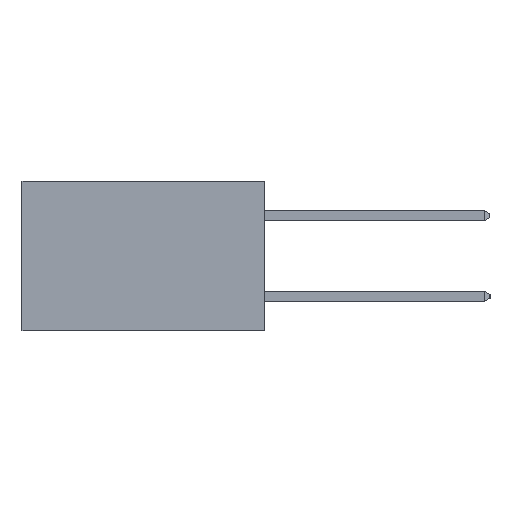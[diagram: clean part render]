
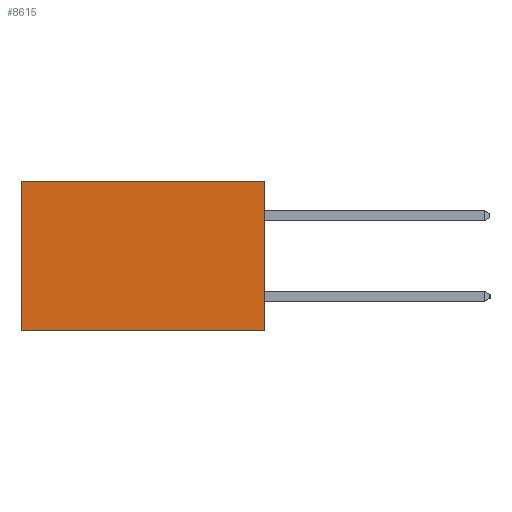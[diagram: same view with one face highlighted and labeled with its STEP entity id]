
A CAD part, left-side view. The second image highlights one B-rep face of the part: STEP entity #8615.
In plain terms, the highlighted planar face has unit normal (-1, 0, 0).
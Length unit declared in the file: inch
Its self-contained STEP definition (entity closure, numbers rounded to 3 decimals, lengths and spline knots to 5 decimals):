
#209 = CARTESIAN_POINT ( 'NONE',  ( 0.2615, 0.6, -0.37 ) ) ;
#807 = CARTESIAN_POINT ( 'NONE',  ( 0.2615, 0.6, -0.37 ) ) ;
#1250 = CARTESIAN_POINT ( 'NONE',  ( 0.2615, 0., -0.37 ) ) ;
#1589 = LINE ( 'NONE', #209, #16834 ) ;
#1616 = ORIENTED_EDGE ( 'NONE', *, *, #17044, .F. ) ;
#1709 = CARTESIAN_POINT ( 'NONE',  ( 0.2615, 0., 0. ) ) ;
#1768 = LINE ( 'NONE', #15288, #12415 ) ;
#2173 = AXIS2_PLACEMENT_3D ( 'NONE', #16874, #16649, #16582 ) ;
#4016 = CARTESIAN_POINT ( 'NONE',  ( 0.2615, 0., -0.37 ) ) ;
#4998 = ORIENTED_EDGE ( 'NONE', *, *, #5314, .F. ) ;
#5011 = VECTOR ( 'NONE', #8431, 39.37008 ) ;
#5314 = EDGE_CURVE ( 'NONE', #8653, #14324, #1768, .T. ) ;
#7022 = VERTEX_POINT ( 'NONE', #1709 ) ;
#7384 = VERTEX_POINT ( 'NONE', #18362 ) ;
#8431 = DIRECTION ( 'NONE',  ( 0., 0., -1. ) ) ;
#8615 = ADVANCED_FACE ( 'NONE', ( #11175 ), #16775, .F. ) ;
#8653 = VERTEX_POINT ( 'NONE', #1250 ) ;
#8899 = DIRECTION ( 'NONE',  ( 0., 1., 0. ) ) ;
#9095 = VECTOR ( 'NONE', #8899, 39.37008 ) ;
#9214 = ORIENTED_EDGE ( 'NONE', *, *, #14606, .T. ) ;
#10471 = DIRECTION ( 'NONE',  ( 0., 0., -1. ) ) ;
#11175 = FACE_OUTER_BOUND ( 'NONE', #14693, .T. ) ;
#11679 = EDGE_CURVE ( 'NONE', #7022, #7384, #13285, .T. ) ;
#12415 = VECTOR ( 'NONE', #15087, 39.37008 ) ;
#13067 = LINE ( 'NONE', #4016, #5011 ) ;
#13150 = CARTESIAN_POINT ( 'NONE',  ( 0.2615, 0., 0. ) ) ;
#13285 = LINE ( 'NONE', #13150, #9095 ) ;
#14324 = VERTEX_POINT ( 'NONE', #807 ) ;
#14606 = EDGE_CURVE ( 'NONE', #7384, #14324, #1589, .T. ) ;
#14693 = EDGE_LOOP ( 'NONE', ( #9214, #4998, #1616, #18443 ) ) ;
#15087 = DIRECTION ( 'NONE',  ( 0., 1., 0. ) ) ;
#15288 = CARTESIAN_POINT ( 'NONE',  ( 0.2615, 0., -0.37 ) ) ;
#16582 = DIRECTION ( 'NONE',  ( 0., 0., -1. ) ) ;
#16649 = DIRECTION ( 'NONE',  ( 1., 0., 0. ) ) ;
#16775 = PLANE ( 'NONE',  #2173 ) ;
#16834 = VECTOR ( 'NONE', #10471, 39.37008 ) ;
#16874 = CARTESIAN_POINT ( 'NONE',  ( 0.2615, 0., -0.37 ) ) ;
#17044 = EDGE_CURVE ( 'NONE', #7022, #8653, #13067, .T. ) ;
#18362 = CARTESIAN_POINT ( 'NONE',  ( 0.2615, 0.6, 0. ) ) ;
#18443 = ORIENTED_EDGE ( 'NONE', *, *, #11679, .T. ) ;
